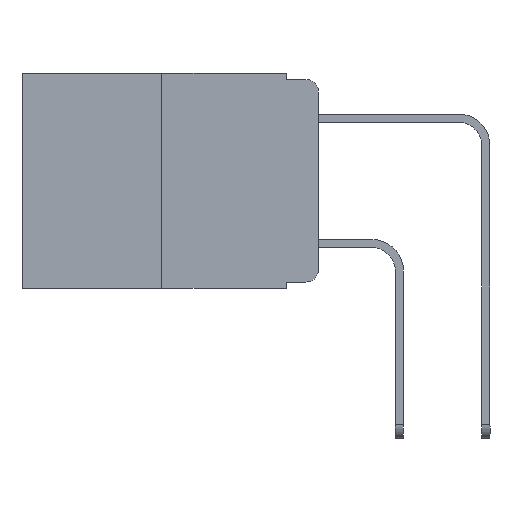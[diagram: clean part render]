
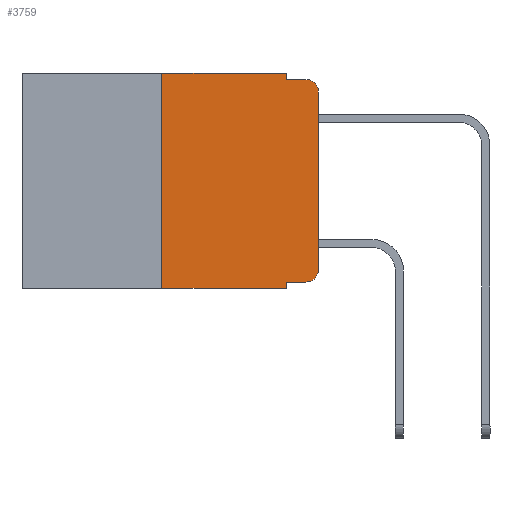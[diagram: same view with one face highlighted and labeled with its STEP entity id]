
A CAD part, left-side view. The second image highlights one B-rep face of the part: STEP entity #3759.
In plain terms, the highlighted planar face has unit normal (-1, 0, 0).
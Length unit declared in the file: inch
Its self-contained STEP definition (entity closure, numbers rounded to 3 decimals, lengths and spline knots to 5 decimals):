
#136 = CARTESIAN_POINT ( 'NONE',  ( 0., 0.051, -0.333 ) ) ;
#555 = CARTESIAN_POINT ( 'NONE',  ( 0., 0.051, -0.333 ) ) ;
#577 = EDGE_CURVE ( 'NONE', #9036, #1274, #3127, .T. ) ;
#641 = EDGE_CURVE ( 'NONE', #12123, #5720, #7127, .T. ) ;
#1077 = LINE ( 'NONE', #136, #10540 ) ;
#1274 = VERTEX_POINT ( 'NONE', #7485 ) ;
#1302 = CARTESIAN_POINT ( 'NONE',  ( 0., 0.473, -0.343 ) ) ;
#1457 = EDGE_CURVE ( 'NONE', #5720, #7841, #8343, .T. ) ;
#1557 = CARTESIAN_POINT ( 'NONE',  ( 0., 0.02, -0.313 ) ) ;
#1606 = EDGE_LOOP ( 'NONE', ( #5873, #12412, #2847, #5739, #3282, #9782, #11615, #2394, #4526, #2145 ) ) ;
#1763 = VECTOR ( 'NONE', #8809, 39.37008 ) ;
#2084 = DIRECTION ( 'NONE',  ( -1., 0., 0. ) ) ;
#2145 = ORIENTED_EDGE ( 'NONE', *, *, #3724, .T. ) ;
#2209 = VERTEX_POINT ( 'NONE', #5714 ) ;
#2394 = ORIENTED_EDGE ( 'NONE', *, *, #7152, .F. ) ;
#2847 = ORIENTED_EDGE ( 'NONE', *, *, #12245, .F. ) ;
#2870 = CARTESIAN_POINT ( 'NONE',  ( 0., 0.473, 0. ) ) ;
#2926 = LINE ( 'NONE', #4678, #9167 ) ;
#3011 = VERTEX_POINT ( 'NONE', #3792 ) ;
#3127 = LINE ( 'NONE', #6939, #11608 ) ;
#3282 = ORIENTED_EDGE ( 'NONE', *, *, #11835, .F. ) ;
#3724 = EDGE_CURVE ( 'NONE', #8788, #12123, #4127, .T. ) ;
#3759 = ADVANCED_FACE ( 'NONE', ( #12284 ), #7569, .F. ) ;
#3792 = CARTESIAN_POINT ( 'NONE',  ( 0., 0.25, 0. ) ) ;
#3866 = CARTESIAN_POINT ( 'NONE',  ( 0., 0.02, -0.01 ) ) ;
#3984 = DIRECTION ( 'NONE',  ( 0., 0., -1. ) ) ;
#3986 = DIRECTION ( 'NONE',  ( 0., -1., 0. ) ) ;
#4127 = CIRCLE ( 'NONE', #11137, 0.02 ) ;
#4526 = ORIENTED_EDGE ( 'NONE', *, *, #10564, .T. ) ;
#4606 = DIRECTION ( 'NONE',  ( 0., 0., 1. ) ) ;
#4678 = CARTESIAN_POINT ( 'NONE',  ( 0., 0.473, 0. ) ) ;
#4857 = CARTESIAN_POINT ( 'NONE',  ( 0., 0.051, 0. ) ) ;
#5128 = DIRECTION ( 'NONE',  ( 0., -1., 0. ) ) ;
#5309 = CARTESIAN_POINT ( 'NONE',  ( 0., 0., 0. ) ) ;
#5639 = DIRECTION ( 'NONE',  ( 0., 0., -1. ) ) ;
#5686 = DIRECTION ( 'NONE',  ( 0., -1., 0. ) ) ;
#5714 = CARTESIAN_POINT ( 'NONE',  ( 0., 0.051, -0.343 ) ) ;
#5720 = VERTEX_POINT ( 'NONE', #9819 ) ;
#5739 = ORIENTED_EDGE ( 'NONE', *, *, #577, .F. ) ;
#5820 = DIRECTION ( 'NONE',  ( 1., 0., 0. ) ) ;
#5873 = ORIENTED_EDGE ( 'NONE', *, *, #641, .T. ) ;
#6131 = CARTESIAN_POINT ( 'NONE',  ( 0., 0.02, -0.333 ) ) ;
#6262 = LINE ( 'NONE', #11929, #9310 ) ;
#6421 = LINE ( 'NONE', #7546, #12340 ) ;
#6939 = CARTESIAN_POINT ( 'NONE',  ( 0., 0.051, 0. ) ) ;
#7127 = LINE ( 'NONE', #5309, #8191 ) ;
#7152 = EDGE_CURVE ( 'NONE', #11344, #2209, #6262, .T. ) ;
#7485 = CARTESIAN_POINT ( 'NONE',  ( 0., 0.051, -0.01 ) ) ;
#7546 = CARTESIAN_POINT ( 'NONE',  ( 0., 0.25, 0. ) ) ;
#7569 = PLANE ( 'NONE',  #9518 ) ;
#7611 = EDGE_CURVE ( 'NONE', #9613, #2209, #9900, .T. ) ;
#7841 = VERTEX_POINT ( 'NONE', #3866 ) ;
#8119 = CARTESIAN_POINT ( 'NONE',  ( 0., 0., -0.313 ) ) ;
#8191 = VECTOR ( 'NONE', #9899, 39.37008 ) ;
#8271 = DIRECTION ( 'NONE',  ( 0., 0., -1. ) ) ;
#8343 = CIRCLE ( 'NONE', #10746, 0.02 ) ;
#8788 = VERTEX_POINT ( 'NONE', #6131 ) ;
#8809 = DIRECTION ( 'NONE',  ( 0., -1., 0. ) ) ;
#8983 = DIRECTION ( 'NONE',  ( 0., 0., -1. ) ) ;
#9036 = VERTEX_POINT ( 'NONE', #4857 ) ;
#9167 = VECTOR ( 'NONE', #5686, 39.37008 ) ;
#9310 = VECTOR ( 'NONE', #8983, 39.37008 ) ;
#9518 = AXIS2_PLACEMENT_3D ( 'NONE', #2870, #5820, #5639 ) ;
#9613 = VERTEX_POINT ( 'NONE', #11691 ) ;
#9677 = LINE ( 'NONE', #10738, #1763 ) ;
#9782 = ORIENTED_EDGE ( 'NONE', *, *, #10392, .F. ) ;
#9819 = CARTESIAN_POINT ( 'NONE',  ( 0., 0., -0.03 ) ) ;
#9899 = DIRECTION ( 'NONE',  ( 0., 0., 1. ) ) ;
#9900 = LINE ( 'NONE', #1302, #9914 ) ;
#9914 = VECTOR ( 'NONE', #5128, 39.37008 ) ;
#10392 = EDGE_CURVE ( 'NONE', #9613, #3011, #6421, .T. ) ;
#10540 = VECTOR ( 'NONE', #3986, 39.37008 ) ;
#10563 = CARTESIAN_POINT ( 'NONE',  ( 0., 0.02, -0.03 ) ) ;
#10564 = EDGE_CURVE ( 'NONE', #11344, #8788, #1077, .T. ) ;
#10738 = CARTESIAN_POINT ( 'NONE',  ( 0., 0.051, -0.01 ) ) ;
#10746 = AXIS2_PLACEMENT_3D ( 'NONE', #10563, #2084, #3984 ) ;
#10777 = DIRECTION ( 'NONE',  ( 0., 0., -1. ) ) ;
#11137 = AXIS2_PLACEMENT_3D ( 'NONE', #1557, #12041, #8271 ) ;
#11344 = VERTEX_POINT ( 'NONE', #555 ) ;
#11608 = VECTOR ( 'NONE', #10777, 39.37008 ) ;
#11615 = ORIENTED_EDGE ( 'NONE', *, *, #7611, .T. ) ;
#11691 = CARTESIAN_POINT ( 'NONE',  ( 0., 0.25, -0.343 ) ) ;
#11835 = EDGE_CURVE ( 'NONE', #3011, #9036, #2926, .T. ) ;
#11929 = CARTESIAN_POINT ( 'NONE',  ( 0., 0.051, 0. ) ) ;
#12041 = DIRECTION ( 'NONE',  ( -1., 0., 0. ) ) ;
#12123 = VERTEX_POINT ( 'NONE', #8119 ) ;
#12245 = EDGE_CURVE ( 'NONE', #1274, #7841, #9677, .T. ) ;
#12284 = FACE_OUTER_BOUND ( 'NONE', #1606, .T. ) ;
#12340 = VECTOR ( 'NONE', #4606, 39.37008 ) ;
#12412 = ORIENTED_EDGE ( 'NONE', *, *, #1457, .T. ) ;
